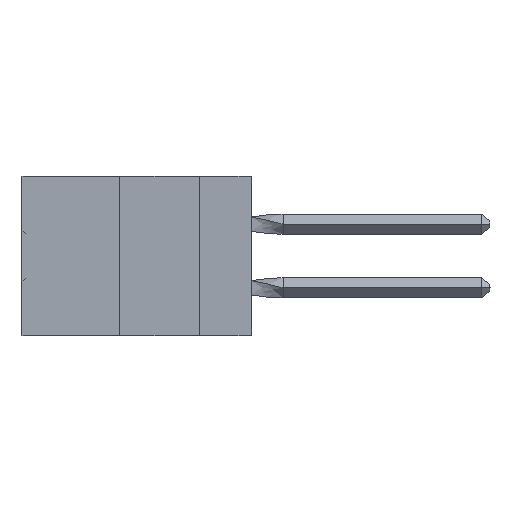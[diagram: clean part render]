
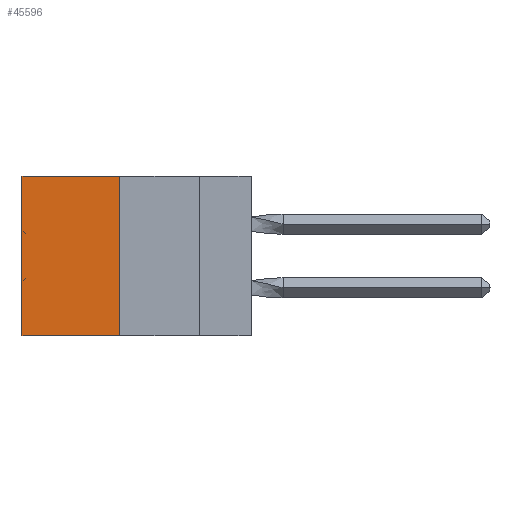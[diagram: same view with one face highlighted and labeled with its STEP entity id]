
A CAD part, left-side view. The second image highlights one B-rep face of the part: STEP entity #45596.
In plain terms, the highlighted planar face has unit normal (-1, 0, 0).
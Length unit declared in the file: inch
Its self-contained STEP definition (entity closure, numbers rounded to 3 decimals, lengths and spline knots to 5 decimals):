
#2193 = ORIENTED_EDGE ( 'NONE', *, *, #2788, .F. ) ;
#2387 = DIRECTION ( 'NONE',  ( 0., 0., -1. ) ) ;
#2788 = EDGE_CURVE ( 'NONE', #39086, #47925, #52022, .T. ) ;
#3884 = CARTESIAN_POINT ( 'NONE',  ( 0.305, 0.413, -0.5 ) ) ;
#5744 = CARTESIAN_POINT ( 'NONE',  ( 0.305, 0.72, 0. ) ) ;
#5835 = VERTEX_POINT ( 'NONE', #23509 ) ;
#6291 = DIRECTION ( 'NONE',  ( 0., 0., -1. ) ) ;
#8268 = DIRECTION ( 'NONE',  ( 0., 0., -1. ) ) ;
#8401 = LINE ( 'NONE', #48196, #38531 ) ;
#11923 = EDGE_CURVE ( 'NONE', #56487, #5835, #38335, .T. ) ;
#13816 = EDGE_LOOP ( 'NONE', ( #38734, #25564, #2193, #38874 ) ) ;
#14237 = VECTOR ( 'NONE', #6291, 39.37008 ) ;
#19596 = EDGE_CURVE ( 'NONE', #47925, #5835, #8401, .T. ) ;
#20320 = VECTOR ( 'NONE', #43851, 39.37008 ) ;
#23509 = CARTESIAN_POINT ( 'NONE',  ( 0.305, 0.72, -0.5 ) ) ;
#23750 = CARTESIAN_POINT ( 'NONE',  ( 0.305, 0.413, -0.5 ) ) ;
#24045 = CARTESIAN_POINT ( 'NONE',  ( 0.305, 0.413, -0.5 ) ) ;
#24417 = DIRECTION ( 'NONE',  ( 1., 0., 0. ) ) ;
#25564 = ORIENTED_EDGE ( 'NONE', *, *, #19596, .F. ) ;
#26406 = CARTESIAN_POINT ( 'NONE',  ( 0.305, 0.413, 0. ) ) ;
#26696 = VECTOR ( 'NONE', #8268, 39.37008 ) ;
#28035 = EDGE_CURVE ( 'NONE', #39086, #56487, #46426, .T. ) ;
#33343 = PLANE ( 'NONE',  #44555 ) ;
#35489 = DIRECTION ( 'NONE',  ( 0., 1., 0. ) ) ;
#35669 = CARTESIAN_POINT ( 'NONE',  ( 0.305, 0.413, 0. ) ) ;
#38335 = LINE ( 'NONE', #56212, #26696 ) ;
#38531 = VECTOR ( 'NONE', #35489, 39.37008 ) ;
#38734 = ORIENTED_EDGE ( 'NONE', *, *, #11923, .T. ) ;
#38874 = ORIENTED_EDGE ( 'NONE', *, *, #28035, .T. ) ;
#39086 = VERTEX_POINT ( 'NONE', #35669 ) ;
#43851 = DIRECTION ( 'NONE',  ( 0., 1., 0. ) ) ;
#44555 = AXIS2_PLACEMENT_3D ( 'NONE', #24045, #24417, #2387 ) ;
#45596 = ADVANCED_FACE ( 'NONE', ( #54157 ), #33343, .F. ) ;
#46426 = LINE ( 'NONE', #26406, #20320 ) ;
#47925 = VERTEX_POINT ( 'NONE', #3884 ) ;
#48196 = CARTESIAN_POINT ( 'NONE',  ( 0.305, 0.413, -0.5 ) ) ;
#52022 = LINE ( 'NONE', #23750, #14237 ) ;
#54157 = FACE_OUTER_BOUND ( 'NONE', #13816, .T. ) ;
#56212 = CARTESIAN_POINT ( 'NONE',  ( 0.305, 0.72, -0.5 ) ) ;
#56487 = VERTEX_POINT ( 'NONE', #5744 ) ;
